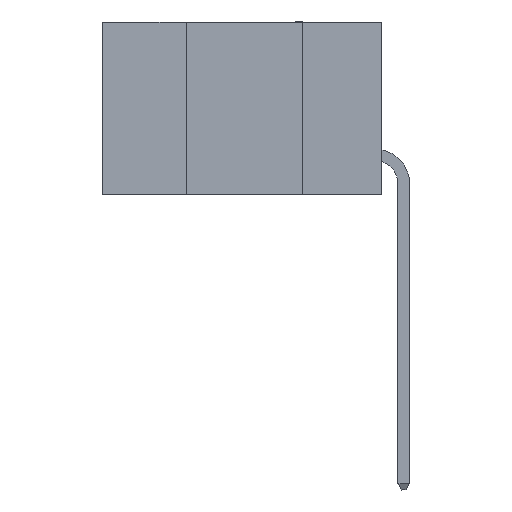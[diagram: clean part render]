
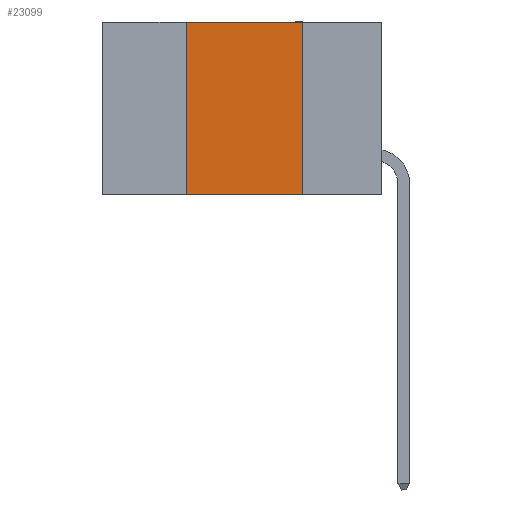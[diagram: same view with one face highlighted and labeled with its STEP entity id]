
A CAD part, left-side view. The second image highlights one B-rep face of the part: STEP entity #23099.
In plain terms, the highlighted planar face has unit normal (-1, 0, 0).
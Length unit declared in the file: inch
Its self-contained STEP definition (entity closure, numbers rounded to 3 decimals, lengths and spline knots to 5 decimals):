
#1184 = CARTESIAN_POINT ( 'NONE',  ( 0., 0.17, -0.37 ) ) ;
#1822 = EDGE_CURVE ( 'NONE', #41209, #9253, #4412, .T. ) ;
#4412 = LINE ( 'NONE', #15818, #28622 ) ;
#6450 = LINE ( 'NONE', #31303, #32740 ) ;
#9253 = VERTEX_POINT ( 'NONE', #1184 ) ;
#9654 = ORIENTED_EDGE ( 'NONE', *, *, #1822, .T. ) ;
#10853 = DIRECTION ( 'NONE',  ( 0., 0., -1. ) ) ;
#13901 = CARTESIAN_POINT ( 'NONE',  ( 0., 0.42, 0. ) ) ;
#13983 = AXIS2_PLACEMENT_3D ( 'NONE', #17697, #37550, #37989 ) ;
#14507 = CARTESIAN_POINT ( 'NONE',  ( 0., 0.17, 0. ) ) ;
#15818 = CARTESIAN_POINT ( 'NONE',  ( 0., 0.6, -0.37 ) ) ;
#16520 = VERTEX_POINT ( 'NONE', #33265 ) ;
#17697 = CARTESIAN_POINT ( 'NONE',  ( 0., 0.6, 0. ) ) ;
#17836 = DIRECTION ( 'NONE',  ( 0., 0., 1. ) ) ;
#23099 = ADVANCED_FACE ( 'NONE', ( #36067 ), #24302, .F. ) ;
#23117 = EDGE_CURVE ( 'NONE', #41209, #16520, #40234, .T. ) ;
#24302 = PLANE ( 'NONE',  #13983 ) ;
#24768 = LINE ( 'NONE', #14507, #41030 ) ;
#26381 = DIRECTION ( 'NONE',  ( 0., -1., 0. ) ) ;
#26850 = CARTESIAN_POINT ( 'NONE',  ( 0., 0.17, 0. ) ) ;
#27387 = ORIENTED_EDGE ( 'NONE', *, *, #23117, .F. ) ;
#28622 = VECTOR ( 'NONE', #26381, 39.37008 ) ;
#28672 = VECTOR ( 'NONE', #17836, 39.37008 ) ;
#31303 = CARTESIAN_POINT ( 'NONE',  ( 0., 0.6, 0. ) ) ;
#32421 = EDGE_CURVE ( 'NONE', #16520, #41089, #6450, .T. ) ;
#32740 = VECTOR ( 'NONE', #34837, 39.37008 ) ;
#33265 = CARTESIAN_POINT ( 'NONE',  ( 0., 0.42, 0. ) ) ;
#33691 = EDGE_LOOP ( 'NONE', ( #36170, #38789, #27387, #9654 ) ) ;
#34837 = DIRECTION ( 'NONE',  ( 0., -1., 0. ) ) ;
#36067 = FACE_OUTER_BOUND ( 'NONE', #33691, .T. ) ;
#36170 = ORIENTED_EDGE ( 'NONE', *, *, #37332, .F. ) ;
#37332 = EDGE_CURVE ( 'NONE', #41089, #9253, #24768, .T. ) ;
#37550 = DIRECTION ( 'NONE',  ( 1., 0., 0. ) ) ;
#37840 = CARTESIAN_POINT ( 'NONE',  ( 0., 0.42, -0.37 ) ) ;
#37989 = DIRECTION ( 'NONE',  ( 0., 0., -1. ) ) ;
#38789 = ORIENTED_EDGE ( 'NONE', *, *, #32421, .F. ) ;
#40234 = LINE ( 'NONE', #13901, #28672 ) ;
#41030 = VECTOR ( 'NONE', #10853, 39.37008 ) ;
#41089 = VERTEX_POINT ( 'NONE', #26850 ) ;
#41209 = VERTEX_POINT ( 'NONE', #37840 ) ;
